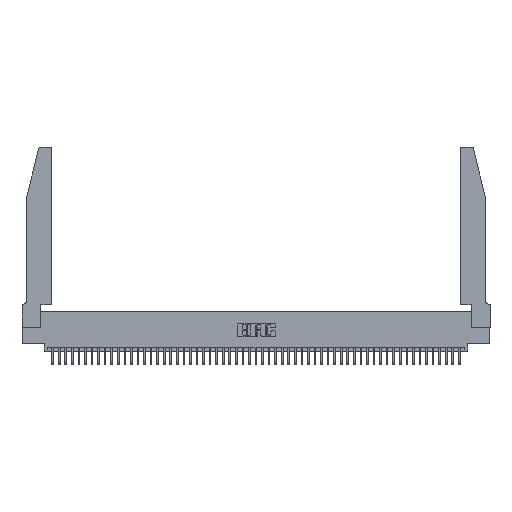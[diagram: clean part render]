
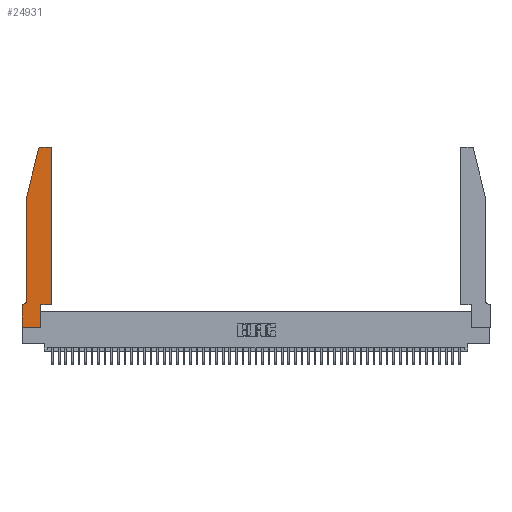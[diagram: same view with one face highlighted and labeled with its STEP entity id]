
A CAD part, top view. The second image highlights one B-rep face of the part: STEP entity #24931.
In plain terms, the highlighted planar face has unit normal (0, 0, 1).
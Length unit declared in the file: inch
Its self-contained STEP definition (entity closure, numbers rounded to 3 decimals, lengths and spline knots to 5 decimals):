
#1049 = DIRECTION ( 'NONE',  ( -0.239, -0.971, 0. ) ) ;
#1454 = CARTESIAN_POINT ( 'NONE',  ( 0.2605, 2.75, 0.37 ) ) ;
#1568 = ORIENTED_EDGE ( 'NONE', *, *, #36173, .T. ) ;
#1622 = EDGE_CURVE ( 'NONE', #40983, #44135, #23574, .T. ) ;
#1672 = CARTESIAN_POINT ( 'NONE',  ( 0., 0., 0.37 ) ) ;
#2459 = CARTESIAN_POINT ( 'NONE',  ( 0.2865, 0.35, 0.37 ) ) ;
#2560 = CARTESIAN_POINT ( 'NONE',  ( 0.4505, 0.35, 0.37 ) ) ;
#3541 = VECTOR ( 'NONE', #8198, 39.37008 ) ;
#3652 = VECTOR ( 'NONE', #51733, 39.37008 ) ;
#4051 = VERTEX_POINT ( 'NONE', #8134 ) ;
#4429 = VECTOR ( 'NONE', #44791, 39.37008 ) ;
#4739 = AXIS2_PLACEMENT_3D ( 'NONE', #14156, #42789, #18309 ) ;
#4768 = DIRECTION ( 'NONE',  ( 0., 0., 1. ) ) ;
#4825 = AXIS2_PLACEMENT_3D ( 'NONE', #29312, #4768, #33424 ) ;
#5409 = CARTESIAN_POINT ( 'NONE',  ( 0., 0., 0.37 ) ) ;
#6681 = VERTEX_POINT ( 'NONE', #16147 ) ;
#7967 = FACE_OUTER_BOUND ( 'NONE', #21725, .T. ) ;
#8134 = CARTESIAN_POINT ( 'NONE',  ( 0.0755, 2., 0.37 ) ) ;
#8198 = DIRECTION ( 'NONE',  ( -1., 0., 0. ) ) ;
#9416 = PLANE ( 'NONE',  #15175 ) ;
#9799 = CARTESIAN_POINT ( 'NONE',  ( 0.284, 2.72, 0.37 ) ) ;
#10627 = ORIENTED_EDGE ( 'NONE', *, *, #10692, .T. ) ;
#10692 = EDGE_CURVE ( 'NONE', #34618, #4051, #50027, .T. ) ;
#11539 = CARTESIAN_POINT ( 'NONE',  ( 0.284, 2.75, 0.37 ) ) ;
#12022 = CIRCLE ( 'NONE', #4739, 0.07 ) ;
#12675 = VECTOR ( 'NONE', #38443, 39.37008 ) ;
#13284 = CARTESIAN_POINT ( 'NONE',  ( 0.4505, 0.35, 0.37 ) ) ;
#13517 = DIRECTION ( 'NONE',  ( 1., 0., 0. ) ) ;
#13915 = DIRECTION ( 'NONE',  ( 1., 0., 0. ) ) ;
#14156 = CARTESIAN_POINT ( 'NONE',  ( 0.0055, 0.42, 0.37 ) ) ;
#14192 = CARTESIAN_POINT ( 'NONE',  ( 0.4205, 2.75, 0.37 ) ) ;
#14453 = ORIENTED_EDGE ( 'NONE', *, *, #25617, .T. ) ;
#14539 = LINE ( 'NONE', #20253, #3541 ) ;
#14561 = ORIENTED_EDGE ( 'NONE', *, *, #40164, .T. ) ;
#15175 = AXIS2_PLACEMENT_3D ( 'NONE', #29753, #38007, #13517 ) ;
#15695 = ORIENTED_EDGE ( 'NONE', *, *, #1622, .T. ) ;
#16067 = VECTOR ( 'NONE', #19003, 39.37008 ) ;
#16147 = CARTESIAN_POINT ( 'NONE',  ( 0.4505, 2.72, 0.37 ) ) ;
#16480 = CARTESIAN_POINT ( 'NONE',  ( 0.0755, 2., 0.37 ) ) ;
#16605 = CIRCLE ( 'NONE', #45103, 0.03 ) ;
#17444 = VECTOR ( 'NONE', #1049, 39.37008 ) ;
#18309 = DIRECTION ( 'NONE',  ( -1., 0., 0. ) ) ;
#19003 = DIRECTION ( 'NONE',  ( 1., 0., 0. ) ) ;
#19025 = VERTEX_POINT ( 'NONE', #35549 ) ;
#20253 = CARTESIAN_POINT ( 'NONE',  ( 0.0755, 0.35, 0.37 ) ) ;
#21725 = EDGE_LOOP ( 'NONE', ( #15695, #25754, #10627, #1568, #32055, #41298, #14561, #46386, #32464, #49403, #37423, #14453 ) ) ;
#21749 = VECTOR ( 'NONE', #34065, 39.37008 ) ;
#23481 = VERTEX_POINT ( 'NONE', #33118 ) ;
#23574 = LINE ( 'NONE', #1454, #12675 ) ;
#24931 = ADVANCED_FACE ( 'NONE', ( #7967 ), #9416, .T. ) ;
#25617 = EDGE_CURVE ( 'NONE', #6681, #40983, #27200, .T. ) ;
#25754 = ORIENTED_EDGE ( 'NONE', *, *, #28988, .T. ) ;
#26746 = VECTOR ( 'NONE', #40978, 39.37008 ) ;
#27200 = CIRCLE ( 'NONE', #4825, 0.03 ) ;
#27207 = CARTESIAN_POINT ( 'NONE',  ( 0.0055, 0.35, 0.37 ) ) ;
#28067 = EDGE_CURVE ( 'NONE', #33892, #6681, #48005, .T. ) ;
#28133 = VECTOR ( 'NONE', #50352, 39.37008 ) ;
#28988 = EDGE_CURVE ( 'NONE', #44135, #34618, #16605, .T. ) ;
#29160 = CARTESIAN_POINT ( 'NONE',  ( 0.2865, 0.35, 0.37 ) ) ;
#29312 = CARTESIAN_POINT ( 'NONE',  ( 0.4205, 2.72, 0.37 ) ) ;
#29753 = CARTESIAN_POINT ( 'NONE',  ( 0., 0.35, 0.37 ) ) ;
#32055 = ORIENTED_EDGE ( 'NONE', *, *, #46513, .T. ) ;
#32388 = CARTESIAN_POINT ( 'NONE',  ( 0.4505, 0.35, 0.37 ) ) ;
#32464 = ORIENTED_EDGE ( 'NONE', *, *, #45974, .T. ) ;
#33118 = CARTESIAN_POINT ( 'NONE',  ( 0.2865, 0., 0.37 ) ) ;
#33424 = DIRECTION ( 'NONE',  ( 1., 0., 0. ) ) ;
#33892 = VERTEX_POINT ( 'NONE', #13284 ) ;
#34065 = DIRECTION ( 'NONE',  ( 1., 0., 0. ) ) ;
#34618 = VERTEX_POINT ( 'NONE', #47526 ) ;
#35549 = CARTESIAN_POINT ( 'NONE',  ( 0.0755, 0.42, 0.37 ) ) ;
#36173 = EDGE_CURVE ( 'NONE', #4051, #19025, #37623, .T. ) ;
#36344 = LINE ( 'NONE', #2459, #3652 ) ;
#36922 = VERTEX_POINT ( 'NONE', #27207 ) ;
#37423 = ORIENTED_EDGE ( 'NONE', *, *, #28067, .T. ) ;
#37623 = LINE ( 'NONE', #16480, #26746 ) ;
#38007 = DIRECTION ( 'NONE',  ( 0., 0., 1. ) ) ;
#38408 = DIRECTION ( 'NONE',  ( 0., 0., 1. ) ) ;
#38443 = DIRECTION ( 'NONE',  ( -1., 0., 0. ) ) ;
#39043 = LINE ( 'NONE', #46281, #28133 ) ;
#39437 = VERTEX_POINT ( 'NONE', #52675 ) ;
#39758 = EDGE_CURVE ( 'NONE', #46309, #33892, #51218, .T. ) ;
#40164 = EDGE_CURVE ( 'NONE', #39437, #51540, #39043, .T. ) ;
#40978 = DIRECTION ( 'NONE',  ( 0., -1., 0. ) ) ;
#40983 = VERTEX_POINT ( 'NONE', #14192 ) ;
#41298 = ORIENTED_EDGE ( 'NONE', *, *, #46892, .T. ) ;
#42789 = DIRECTION ( 'NONE',  ( 0., 0., -1. ) ) ;
#44135 = VERTEX_POINT ( 'NONE', #11539 ) ;
#44791 = DIRECTION ( 'NONE',  ( 0., 1., 0. ) ) ;
#45103 = AXIS2_PLACEMENT_3D ( 'NONE', #9799, #38408, #13915 ) ;
#45974 = EDGE_CURVE ( 'NONE', #23481, #46309, #36344, .T. ) ;
#46281 = CARTESIAN_POINT ( 'NONE',  ( 0., 0., 0.37 ) ) ;
#46309 = VERTEX_POINT ( 'NONE', #29160 ) ;
#46386 = ORIENTED_EDGE ( 'NONE', *, *, #52704, .T. ) ;
#46513 = EDGE_CURVE ( 'NONE', #19025, #36922, #12022, .T. ) ;
#46892 = EDGE_CURVE ( 'NONE', #36922, #39437, #14539, .T. ) ;
#47526 = CARTESIAN_POINT ( 'NONE',  ( 0.25487, 2.72718, 0.37 ) ) ;
#48005 = LINE ( 'NONE', #32388, #4429 ) ;
#49403 = ORIENTED_EDGE ( 'NONE', *, *, #39758, .T. ) ;
#50027 = LINE ( 'NONE', #50197, #17444 ) ;
#50197 = CARTESIAN_POINT ( 'NONE',  ( 0.0755, 2., 0.37 ) ) ;
#50352 = DIRECTION ( 'NONE',  ( 0., -1., 0. ) ) ;
#51218 = LINE ( 'NONE', #2560, #16067 ) ;
#51540 = VERTEX_POINT ( 'NONE', #1672 ) ;
#51733 = DIRECTION ( 'NONE',  ( 0., 1., 0. ) ) ;
#51738 = LINE ( 'NONE', #5409, #21749 ) ;
#52675 = CARTESIAN_POINT ( 'NONE',  ( 0., 0.35, 0.37 ) ) ;
#52704 = EDGE_CURVE ( 'NONE', #51540, #23481, #51738, .T. ) ;
